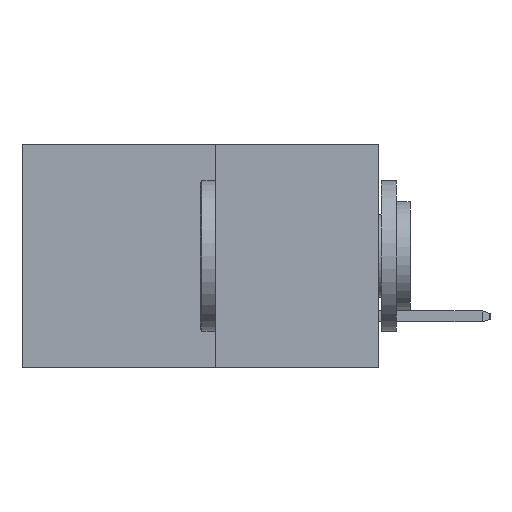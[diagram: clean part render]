
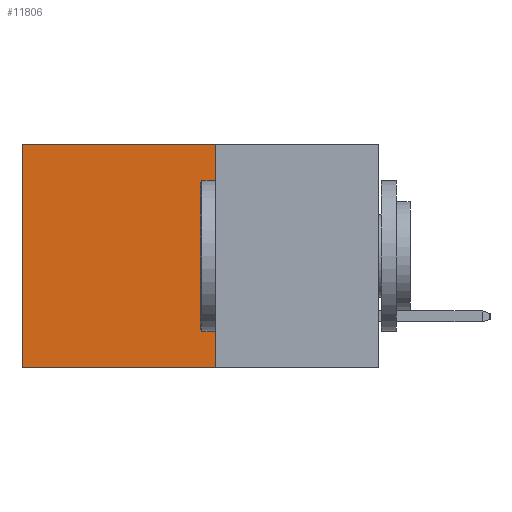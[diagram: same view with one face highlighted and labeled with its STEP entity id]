
A CAD part, left-side view. The second image highlights one B-rep face of the part: STEP entity #11806.
In plain terms, the highlighted planar face has unit normal (-1, 0, 0).
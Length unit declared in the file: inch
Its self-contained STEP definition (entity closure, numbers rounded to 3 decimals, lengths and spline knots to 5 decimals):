
#25 = VERTEX_POINT ( 'NONE', #11160 ) ;
#689 = EDGE_LOOP ( 'NONE', ( #6326, #4691, #11544, #14098 ) ) ;
#1702 = CARTESIAN_POINT ( 'NONE',  ( 0.277, 0.27, 0. ) ) ;
#2724 = CARTESIAN_POINT ( 'NONE',  ( 0.277, 0.27, -0.37 ) ) ;
#3241 = DIRECTION ( 'NONE',  ( 0., 0., -1. ) ) ;
#3330 = LINE ( 'NONE', #10313, #6875 ) ;
#3682 = CARTESIAN_POINT ( 'NONE',  ( 0.277, 0.27, -0.37 ) ) ;
#3949 = DIRECTION ( 'NONE',  ( 0., 0., -1. ) ) ;
#3953 = VECTOR ( 'NONE', #9271, 39.37008 ) ;
#4365 = VERTEX_POINT ( 'NONE', #11887 ) ;
#4691 = ORIENTED_EDGE ( 'NONE', *, *, #8638, .F. ) ;
#6317 = LINE ( 'NONE', #3682, #9402 ) ;
#6326 = ORIENTED_EDGE ( 'NONE', *, *, #8410, .T. ) ;
#6597 = EDGE_CURVE ( 'NONE', #14124, #4365, #7085, .T. ) ;
#6875 = VECTOR ( 'NONE', #3241, 39.37008 ) ;
#7085 = LINE ( 'NONE', #9432, #3953 ) ;
#8410 = EDGE_CURVE ( 'NONE', #25, #14810, #3330, .T. ) ;
#8608 = PLANE ( 'NONE',  #14223 ) ;
#8638 = EDGE_CURVE ( 'NONE', #4365, #14810, #6317, .T. ) ;
#8815 = CARTESIAN_POINT ( 'NONE',  ( 0.277, 0.27, 0. ) ) ;
#9271 = DIRECTION ( 'NONE',  ( 0., 0., -1. ) ) ;
#9402 = VECTOR ( 'NONE', #13026, 39.37008 ) ;
#9432 = CARTESIAN_POINT ( 'NONE',  ( 0.277, 0.27, -0.37 ) ) ;
#10313 = CARTESIAN_POINT ( 'NONE',  ( 0.277, 0.59, -0.37 ) ) ;
#10959 = DIRECTION ( 'NONE',  ( 1., 0., 0. ) ) ;
#11160 = CARTESIAN_POINT ( 'NONE',  ( 0.277, 0.59, 0. ) ) ;
#11349 = CARTESIAN_POINT ( 'NONE',  ( 0.277, 0.59, -0.37 ) ) ;
#11544 = ORIENTED_EDGE ( 'NONE', *, *, #6597, .F. ) ;
#11647 = LINE ( 'NONE', #1702, #13627 ) ;
#11806 = ADVANCED_FACE ( 'NONE', ( #14390 ), #8608, .F. ) ;
#11887 = CARTESIAN_POINT ( 'NONE',  ( 0.277, 0.27, -0.37 ) ) ;
#13026 = DIRECTION ( 'NONE',  ( 0., 1., 0. ) ) ;
#13627 = VECTOR ( 'NONE', #14530, 39.37008 ) ;
#14098 = ORIENTED_EDGE ( 'NONE', *, *, #14681, .T. ) ;
#14124 = VERTEX_POINT ( 'NONE', #8815 ) ;
#14223 = AXIS2_PLACEMENT_3D ( 'NONE', #2724, #10959, #3949 ) ;
#14390 = FACE_OUTER_BOUND ( 'NONE', #689, .T. ) ;
#14530 = DIRECTION ( 'NONE',  ( 0., 1., 0. ) ) ;
#14681 = EDGE_CURVE ( 'NONE', #14124, #25, #11647, .T. ) ;
#14810 = VERTEX_POINT ( 'NONE', #11349 ) ;
